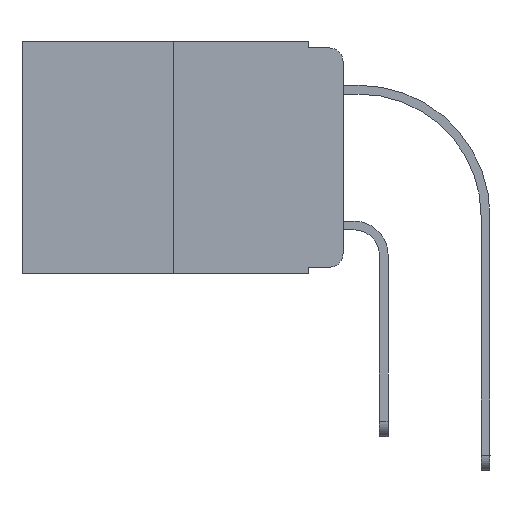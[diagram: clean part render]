
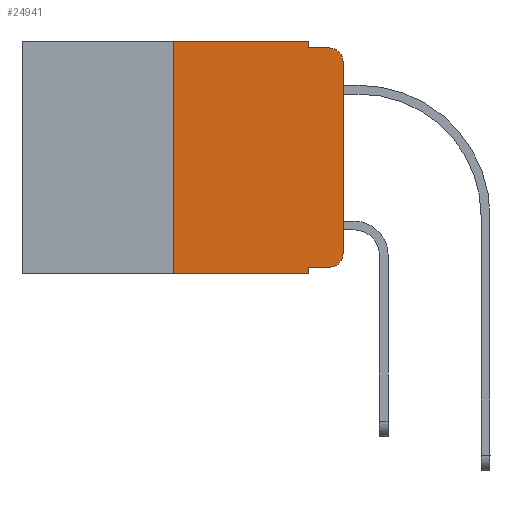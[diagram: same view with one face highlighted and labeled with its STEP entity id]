
A CAD part, left-side view. The second image highlights one B-rep face of the part: STEP entity #24941.
In plain terms, the highlighted planar face has unit normal (-1, 0, 0).
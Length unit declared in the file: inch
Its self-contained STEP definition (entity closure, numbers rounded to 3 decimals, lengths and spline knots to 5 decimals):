
#1026 = CARTESIAN_POINT ( 'NONE',  ( 0., 0.473, 0. ) ) ;
#1155 = LINE ( 'NONE', #5201, #9957 ) ;
#1238 = VECTOR ( 'NONE', #16060, 39.37008 ) ;
#1472 = VECTOR ( 'NONE', #23077, 39.37008 ) ;
#1496 = CARTESIAN_POINT ( 'NONE',  ( 0., 0.051, -0.343 ) ) ;
#2211 = EDGE_CURVE ( 'NONE', #5219, #24148, #23142, .T. ) ;
#2229 = CIRCLE ( 'NONE', #5577, 0.02 ) ;
#2414 = ORIENTED_EDGE ( 'NONE', *, *, #8224, .T. ) ;
#2444 = CARTESIAN_POINT ( 'NONE',  ( 0., 0., -0.313 ) ) ;
#2850 = DIRECTION ( 'NONE',  ( 0., 0., -1. ) ) ;
#2902 = EDGE_CURVE ( 'NONE', #20866, #24148, #6207, .T. ) ;
#2982 = DIRECTION ( 'NONE',  ( 1., 0., 0. ) ) ;
#3907 = VECTOR ( 'NONE', #12796, 39.37008 ) ;
#4897 = DIRECTION ( 'NONE',  ( 0., 0., -1. ) ) ;
#5096 = CARTESIAN_POINT ( 'NONE',  ( 0., 0.473, -0.343 ) ) ;
#5201 = CARTESIAN_POINT ( 'NONE',  ( 0., 0.051, -0.333 ) ) ;
#5219 = VERTEX_POINT ( 'NONE', #22331 ) ;
#5238 = ORIENTED_EDGE ( 'NONE', *, *, #17394, .F. ) ;
#5577 = AXIS2_PLACEMENT_3D ( 'NONE', #12162, #12299, #14251 ) ;
#6207 = LINE ( 'NONE', #9729, #23932 ) ;
#6410 = EDGE_CURVE ( 'NONE', #7134, #16950, #16067, .T. ) ;
#6930 = CARTESIAN_POINT ( 'NONE',  ( 0., 0., 0. ) ) ;
#6934 = LINE ( 'NONE', #5096, #3907 ) ;
#7072 = ORIENTED_EDGE ( 'NONE', *, *, #12093, .T. ) ;
#7111 = DIRECTION ( 'NONE',  ( -1., 0., 0. ) ) ;
#7134 = VERTEX_POINT ( 'NONE', #24368 ) ;
#7297 = AXIS2_PLACEMENT_3D ( 'NONE', #25006, #7111, #15056 ) ;
#8121 = CARTESIAN_POINT ( 'NONE',  ( 0., 0.051, 0. ) ) ;
#8224 = EDGE_CURVE ( 'NONE', #15862, #5219, #19072, .T. ) ;
#8570 = EDGE_CURVE ( 'NONE', #16276, #17460, #1155, .T. ) ;
#9033 = ORIENTED_EDGE ( 'NONE', *, *, #2902, .F. ) ;
#9729 = CARTESIAN_POINT ( 'NONE',  ( 0., 0.051, -0.01 ) ) ;
#9957 = VECTOR ( 'NONE', #15100, 39.37008 ) ;
#10308 = ORIENTED_EDGE ( 'NONE', *, *, #17870, .T. ) ;
#10538 = VERTEX_POINT ( 'NONE', #13519 ) ;
#10916 = LINE ( 'NONE', #1026, #1472 ) ;
#12093 = EDGE_CURVE ( 'NONE', #7134, #14884, #6934, .T. ) ;
#12162 = CARTESIAN_POINT ( 'NONE',  ( 0., 0.02, -0.313 ) ) ;
#12299 = DIRECTION ( 'NONE',  ( -1., 0., 0. ) ) ;
#12485 = AXIS2_PLACEMENT_3D ( 'NONE', #13169, #2982, #2850 ) ;
#12673 = LINE ( 'NONE', #8121, #1238 ) ;
#12796 = DIRECTION ( 'NONE',  ( 0., -1., 0. ) ) ;
#12899 = PLANE ( 'NONE',  #12485 ) ;
#12914 = CARTESIAN_POINT ( 'NONE',  ( 0., 0.25, 0. ) ) ;
#13169 = CARTESIAN_POINT ( 'NONE',  ( 0., 0.473, 0. ) ) ;
#13519 = CARTESIAN_POINT ( 'NONE',  ( 0., 0.051, 0. ) ) ;
#13774 = CARTESIAN_POINT ( 'NONE',  ( 0., 0.02, -0.333 ) ) ;
#14251 = DIRECTION ( 'NONE',  ( 0., 0., -1. ) ) ;
#14882 = DIRECTION ( 'NONE',  ( 0., 0., 1. ) ) ;
#14884 = VERTEX_POINT ( 'NONE', #1496 ) ;
#15056 = DIRECTION ( 'NONE',  ( 0., 0., -1. ) ) ;
#15100 = DIRECTION ( 'NONE',  ( 0., -1., 0. ) ) ;
#15862 = VERTEX_POINT ( 'NONE', #2444 ) ;
#16060 = DIRECTION ( 'NONE',  ( 0., 0., -1. ) ) ;
#16067 = LINE ( 'NONE', #17784, #16153 ) ;
#16153 = VECTOR ( 'NONE', #21838, 39.37008 ) ;
#16276 = VERTEX_POINT ( 'NONE', #23710 ) ;
#16950 = VERTEX_POINT ( 'NONE', #12914 ) ;
#17394 = EDGE_CURVE ( 'NONE', #16950, #10538, #10916, .T. ) ;
#17460 = VERTEX_POINT ( 'NONE', #13774 ) ;
#17784 = CARTESIAN_POINT ( 'NONE',  ( 0., 0.25, 0. ) ) ;
#17870 = EDGE_CURVE ( 'NONE', #17460, #15862, #2229, .T. ) ;
#17897 = CARTESIAN_POINT ( 'NONE',  ( 0., 0.02, -0.01 ) ) ;
#18996 = EDGE_CURVE ( 'NONE', #16276, #14884, #19010, .T. ) ;
#19010 = LINE ( 'NONE', #25262, #23566 ) ;
#19072 = LINE ( 'NONE', #6930, #25393 ) ;
#19304 = EDGE_LOOP ( 'NONE', ( #2414, #25489, #9033, #20518, #5238, #23461, #7072, #21664, #24816, #10308 ) ) ;
#20046 = DIRECTION ( 'NONE',  ( 0., -1., 0. ) ) ;
#20518 = ORIENTED_EDGE ( 'NONE', *, *, #24443, .F. ) ;
#20866 = VERTEX_POINT ( 'NONE', #25315 ) ;
#20885 = FACE_OUTER_BOUND ( 'NONE', #19304, .T. ) ;
#21664 = ORIENTED_EDGE ( 'NONE', *, *, #18996, .F. ) ;
#21838 = DIRECTION ( 'NONE',  ( 0., 0., 1. ) ) ;
#22331 = CARTESIAN_POINT ( 'NONE',  ( 0., 0., -0.03 ) ) ;
#23077 = DIRECTION ( 'NONE',  ( 0., -1., 0. ) ) ;
#23142 = CIRCLE ( 'NONE', #7297, 0.02 ) ;
#23461 = ORIENTED_EDGE ( 'NONE', *, *, #6410, .F. ) ;
#23566 = VECTOR ( 'NONE', #4897, 39.37008 ) ;
#23710 = CARTESIAN_POINT ( 'NONE',  ( 0., 0.051, -0.333 ) ) ;
#23932 = VECTOR ( 'NONE', #20046, 39.37008 ) ;
#24148 = VERTEX_POINT ( 'NONE', #17897 ) ;
#24368 = CARTESIAN_POINT ( 'NONE',  ( 0., 0.25, -0.343 ) ) ;
#24443 = EDGE_CURVE ( 'NONE', #10538, #20866, #12673, .T. ) ;
#24816 = ORIENTED_EDGE ( 'NONE', *, *, #8570, .T. ) ;
#24941 = ADVANCED_FACE ( 'NONE', ( #20885 ), #12899, .F. ) ;
#25006 = CARTESIAN_POINT ( 'NONE',  ( 0., 0.02, -0.03 ) ) ;
#25262 = CARTESIAN_POINT ( 'NONE',  ( 0., 0.051, 0. ) ) ;
#25315 = CARTESIAN_POINT ( 'NONE',  ( 0., 0.051, -0.01 ) ) ;
#25393 = VECTOR ( 'NONE', #14882, 39.37008 ) ;
#25489 = ORIENTED_EDGE ( 'NONE', *, *, #2211, .T. ) ;
